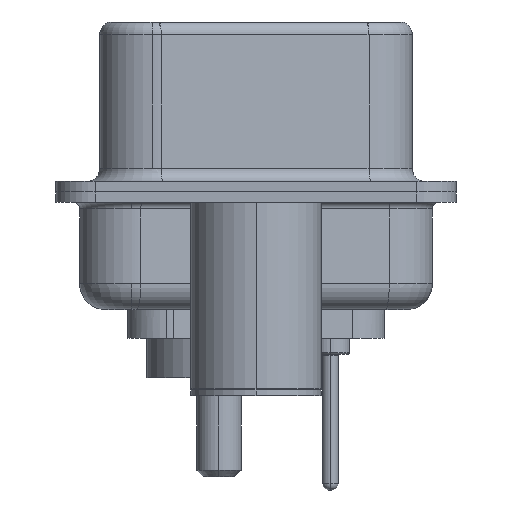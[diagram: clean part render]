
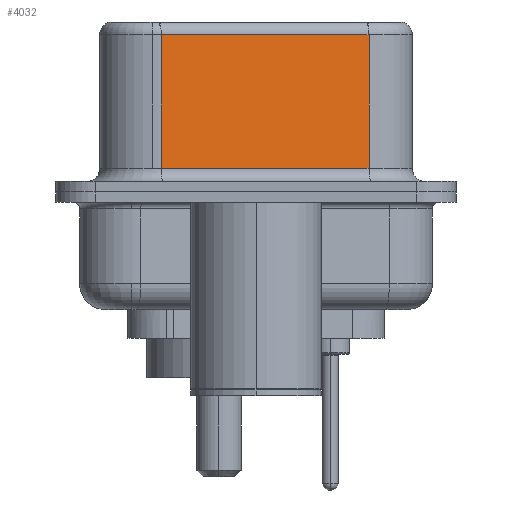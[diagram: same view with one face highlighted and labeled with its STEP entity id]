
A CAD part, left-side view. The second image highlights one B-rep face of the part: STEP entity #4032.
In plain terms, the highlighted planar face has unit normal (-0.985, -0.174, 0).
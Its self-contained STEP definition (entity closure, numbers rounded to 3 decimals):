
#402 = VERTEX_POINT ( 'NONE', #17026 ) ;
#627 = EDGE_LOOP ( 'NONE', ( #17451, #21912, #21944, #16808 ) ) ;
#2585 = LINE ( 'NONE', #10310, #22293 ) ;
#4032 = ADVANCED_FACE ( 'NONE', ( #13475 ), #24217, .F. ) ;
#4315 = VERTEX_POINT ( 'NONE', #16391 ) ;
#4841 = EDGE_CURVE ( 'NONE', #7248, #15211, #2585, .T. ) ;
#5085 = DIRECTION ( 'NONE',  ( 0.174, -0.985, 0. ) ) ;
#6994 = EDGE_CURVE ( 'NONE', #402, #4315, #22153, .T. ) ;
#7093 = DIRECTION ( 'NONE',  ( -0.174, 0.985, 0. ) ) ;
#7108 = EDGE_CURVE ( 'NONE', #15211, #4315, #19751, .T. ) ;
#7248 = VERTEX_POINT ( 'NONE', #11423 ) ;
#7368 = DIRECTION ( 'NONE',  ( -0.174, 0.985, 0. ) ) ;
#7958 = VECTOR ( 'NONE', #7093, 1000. ) ;
#9087 = CARTESIAN_POINT ( 'NONE',  ( 5.132, -4.322, 6.52 ) ) ;
#10310 = CARTESIAN_POINT ( 'NONE',  ( 3.73, 3.628, 6.52 ) ) ;
#11423 = CARTESIAN_POINT ( 'NONE',  ( 3.73, 3.628, 6.02 ) ) ;
#11489 = DIRECTION ( 'NONE',  ( 0., 0., -1. ) ) ;
#12734 = DIRECTION ( 'NONE',  ( 0., 0., -1. ) ) ;
#13475 = FACE_OUTER_BOUND ( 'NONE', #627, .T. ) ;
#14523 = VECTOR ( 'NONE', #5085, 1000. ) ;
#15211 = VERTEX_POINT ( 'NONE', #22627 ) ;
#16365 = VECTOR ( 'NONE', #12734, 1000. ) ;
#16391 = CARTESIAN_POINT ( 'NONE',  ( 5.132, -4.322, 0.9 ) ) ;
#16808 = ORIENTED_EDGE ( 'NONE', *, *, #7108, .T. ) ;
#17026 = CARTESIAN_POINT ( 'NONE',  ( 5.132, -4.322, 6.02 ) ) ;
#17451 = ORIENTED_EDGE ( 'NONE', *, *, #6994, .F. ) ;
#18544 = LINE ( 'NONE', #18970, #7958 ) ;
#18950 = CARTESIAN_POINT ( 'NONE',  ( 5.132, -4.322, 0.9 ) ) ;
#18970 = CARTESIAN_POINT ( 'NONE',  ( 5.132, -4.322, 6.02 ) ) ;
#19234 = DIRECTION ( 'NONE',  ( 0.985, 0.174, 0. ) ) ;
#19751 = LINE ( 'NONE', #18950, #14523 ) ;
#19876 = EDGE_CURVE ( 'NONE', #402, #7248, #18544, .T. ) ;
#20188 = AXIS2_PLACEMENT_3D ( 'NONE', #9087, #19234, #7368 ) ;
#21912 = ORIENTED_EDGE ( 'NONE', *, *, #19876, .T. ) ;
#21944 = ORIENTED_EDGE ( 'NONE', *, *, #4841, .T. ) ;
#22153 = LINE ( 'NONE', #22487, #16365 ) ;
#22293 = VECTOR ( 'NONE', #11489, 1000. ) ;
#22487 = CARTESIAN_POINT ( 'NONE',  ( 5.132, -4.322, 6.52 ) ) ;
#22627 = CARTESIAN_POINT ( 'NONE',  ( 3.73, 3.628, 0.9 ) ) ;
#24217 = PLANE ( 'NONE',  #20188 ) ;
